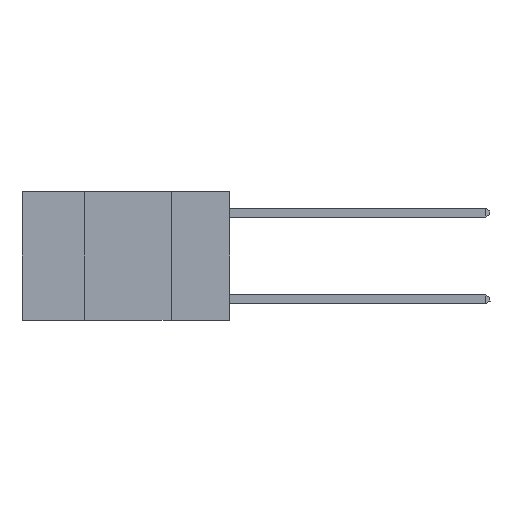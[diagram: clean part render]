
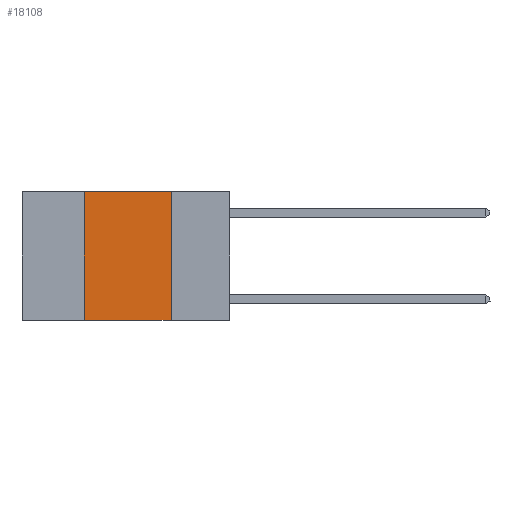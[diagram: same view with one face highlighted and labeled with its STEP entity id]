
A CAD part, left-side view. The second image highlights one B-rep face of the part: STEP entity #18108.
In plain terms, the highlighted planar face has unit normal (-1, 0, 0).
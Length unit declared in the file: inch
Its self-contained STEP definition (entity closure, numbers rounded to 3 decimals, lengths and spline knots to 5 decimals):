
#594 = EDGE_CURVE ( 'NONE', #19367, #10077, #9437, .T. ) ;
#2283 = DIRECTION ( 'NONE',  ( 0., -1., 0. ) ) ;
#2592 = CARTESIAN_POINT ( 'NONE',  ( 0., 0.42, 0. ) ) ;
#2711 = EDGE_CURVE ( 'NONE', #19412, #19010, #19783, .T. ) ;
#4345 = LINE ( 'NONE', #17195, #15865 ) ;
#5136 = CARTESIAN_POINT ( 'NONE',  ( 0., 0.17, -0.37 ) ) ;
#5229 = DIRECTION ( 'NONE',  ( 0., -1., 0. ) ) ;
#5477 = CARTESIAN_POINT ( 'NONE',  ( 0., 0.6, 0. ) ) ;
#6810 = EDGE_CURVE ( 'NONE', #10077, #19412, #18371, .T. ) ;
#7584 = EDGE_LOOP ( 'NONE', ( #11515, #15977, #9041, #12906 ) ) ;
#8545 = DIRECTION ( 'NONE',  ( 1., 0., 0. ) ) ;
#8779 = DIRECTION ( 'NONE',  ( 0., 0., 1. ) ) ;
#9041 = ORIENTED_EDGE ( 'NONE', *, *, #594, .F. ) ;
#9437 = LINE ( 'NONE', #2592, #16898 ) ;
#10077 = VERTEX_POINT ( 'NONE', #11920 ) ;
#11346 = CARTESIAN_POINT ( 'NONE',  ( 0., 0.6, 0. ) ) ;
#11515 = ORIENTED_EDGE ( 'NONE', *, *, #2711, .F. ) ;
#11920 = CARTESIAN_POINT ( 'NONE',  ( 0., 0.42, 0. ) ) ;
#12861 = FACE_OUTER_BOUND ( 'NONE', #7584, .T. ) ;
#12906 = ORIENTED_EDGE ( 'NONE', *, *, #19392, .T. ) ;
#14056 = CARTESIAN_POINT ( 'NONE',  ( 0., 0.42, -0.37 ) ) ;
#14549 = DIRECTION ( 'NONE',  ( 0., 0., -1. ) ) ;
#15677 = CARTESIAN_POINT ( 'NONE',  ( 0., 0.17, 0. ) ) ;
#15865 = VECTOR ( 'NONE', #5229, 39.37008 ) ;
#15977 = ORIENTED_EDGE ( 'NONE', *, *, #6810, .F. ) ;
#16297 = CARTESIAN_POINT ( 'NONE',  ( 0., 0.17, 0. ) ) ;
#16898 = VECTOR ( 'NONE', #8779, 39.37008 ) ;
#17195 = CARTESIAN_POINT ( 'NONE',  ( 0., 0.6, -0.37 ) ) ;
#17489 = PLANE ( 'NONE',  #17689 ) ;
#17689 = AXIS2_PLACEMENT_3D ( 'NONE', #5477, #8545, #19082 ) ;
#17881 = VECTOR ( 'NONE', #2283, 39.37008 ) ;
#18108 = ADVANCED_FACE ( 'NONE', ( #12861 ), #17489, .F. ) ;
#18371 = LINE ( 'NONE', #11346, #17881 ) ;
#19010 = VERTEX_POINT ( 'NONE', #5136 ) ;
#19082 = DIRECTION ( 'NONE',  ( 0., 0., -1. ) ) ;
#19277 = VECTOR ( 'NONE', #14549, 39.37008 ) ;
#19367 = VERTEX_POINT ( 'NONE', #14056 ) ;
#19392 = EDGE_CURVE ( 'NONE', #19367, #19010, #4345, .T. ) ;
#19412 = VERTEX_POINT ( 'NONE', #15677 ) ;
#19783 = LINE ( 'NONE', #16297, #19277 ) ;
